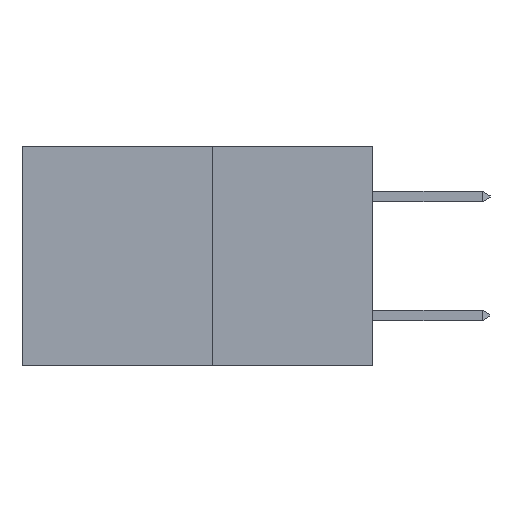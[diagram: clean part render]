
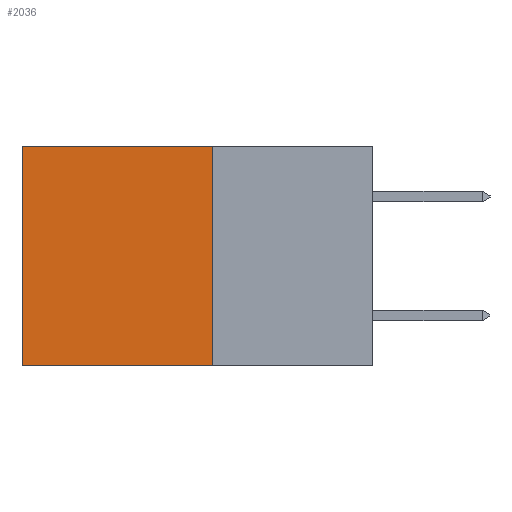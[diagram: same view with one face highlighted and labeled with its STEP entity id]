
A CAD part, left-side view. The second image highlights one B-rep face of the part: STEP entity #2036.
In plain terms, the highlighted planar face has unit normal (-1, 0, 0).
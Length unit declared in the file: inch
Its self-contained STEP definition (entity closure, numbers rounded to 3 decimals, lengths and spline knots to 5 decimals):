
#14 = ORIENTED_EDGE ( 'NONE', *, *, #6302, .F. ) ;
#305 = DIRECTION ( 'NONE',  ( 0., 0., -1. ) ) ;
#803 = AXIS2_PLACEMENT_3D ( 'NONE', #11321, #9572, #6906 ) ;
#1685 = VERTEX_POINT ( 'NONE', #11074 ) ;
#1936 = VERTEX_POINT ( 'NONE', #9515 ) ;
#2036 = ADVANCED_FACE ( 'NONE', ( #12224 ), #9161, .F. ) ;
#2226 = LINE ( 'NONE', #4506, #9165 ) ;
#2307 = CARTESIAN_POINT ( 'NONE',  ( 0.277, 0.27, 0. ) ) ;
#2459 = VECTOR ( 'NONE', #10721, 39.37008 ) ;
#2586 = EDGE_CURVE ( 'NONE', #1685, #1936, #2226, .T. ) ;
#2670 = LINE ( 'NONE', #6435, #9838 ) ;
#3373 = VERTEX_POINT ( 'NONE', #2307 ) ;
#3650 = DIRECTION ( 'NONE',  ( 0., 1., 0. ) ) ;
#3676 = CARTESIAN_POINT ( 'NONE',  ( 0.277, 0.27, 0. ) ) ;
#4023 = ORIENTED_EDGE ( 'NONE', *, *, #2586, .T. ) ;
#4078 = EDGE_CURVE ( 'NONE', #4825, #1936, #2670, .T. ) ;
#4279 = EDGE_CURVE ( 'NONE', #3373, #1685, #8440, .T. ) ;
#4506 = CARTESIAN_POINT ( 'NONE',  ( 0.277, 0.59, -0.37 ) ) ;
#4825 = VERTEX_POINT ( 'NONE', #10399 ) ;
#5026 = LINE ( 'NONE', #10759, #2459 ) ;
#5690 = VECTOR ( 'NONE', #3650, 39.37008 ) ;
#6302 = EDGE_CURVE ( 'NONE', #3373, #4825, #5026, .T. ) ;
#6435 = CARTESIAN_POINT ( 'NONE',  ( 0.277, 0.27, -0.37 ) ) ;
#6447 = DIRECTION ( 'NONE',  ( 0., 1., 0. ) ) ;
#6906 = DIRECTION ( 'NONE',  ( 0., 0., -1. ) ) ;
#6988 = ORIENTED_EDGE ( 'NONE', *, *, #4078, .F. ) ;
#7430 = ORIENTED_EDGE ( 'NONE', *, *, #4279, .T. ) ;
#8440 = LINE ( 'NONE', #3676, #5690 ) ;
#9161 = PLANE ( 'NONE',  #803 ) ;
#9165 = VECTOR ( 'NONE', #305, 39.37008 ) ;
#9515 = CARTESIAN_POINT ( 'NONE',  ( 0.277, 0.59, -0.37 ) ) ;
#9572 = DIRECTION ( 'NONE',  ( 1., 0., 0. ) ) ;
#9838 = VECTOR ( 'NONE', #6447, 39.37008 ) ;
#10399 = CARTESIAN_POINT ( 'NONE',  ( 0.277, 0.27, -0.37 ) ) ;
#10721 = DIRECTION ( 'NONE',  ( 0., 0., -1. ) ) ;
#10759 = CARTESIAN_POINT ( 'NONE',  ( 0.277, 0.27, -0.37 ) ) ;
#11074 = CARTESIAN_POINT ( 'NONE',  ( 0.277, 0.59, 0. ) ) ;
#11321 = CARTESIAN_POINT ( 'NONE',  ( 0.277, 0.27, -0.37 ) ) ;
#11982 = EDGE_LOOP ( 'NONE', ( #4023, #6988, #14, #7430 ) ) ;
#12224 = FACE_OUTER_BOUND ( 'NONE', #11982, .T. ) ;
